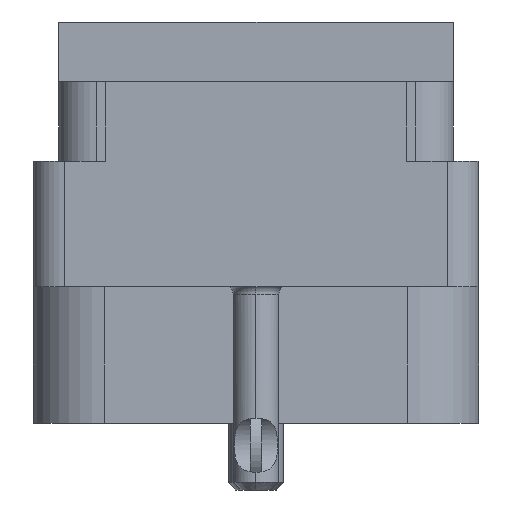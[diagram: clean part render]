
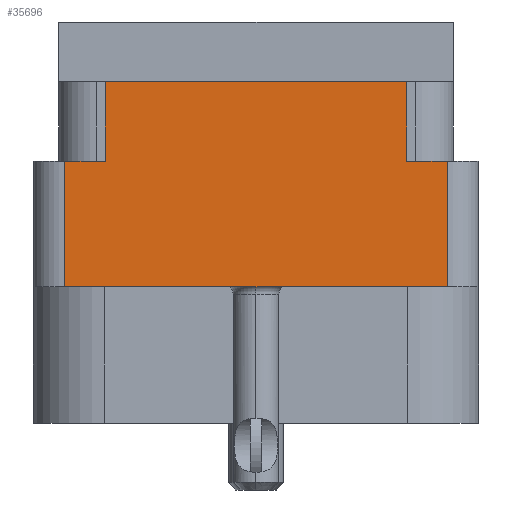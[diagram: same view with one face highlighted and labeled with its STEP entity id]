
A CAD part, left-side view. The second image highlights one B-rep face of the part: STEP entity #35696.
In plain terms, the highlighted planar face has unit normal (-1, 0, 0).
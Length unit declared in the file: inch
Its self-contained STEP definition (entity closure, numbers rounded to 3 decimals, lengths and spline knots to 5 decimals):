
#318 = DIRECTION ( 'NONE',  ( 0., -1., 0. ) ) ;
#1235 = PLANE ( 'NONE',  #37064 ) ;
#1629 = VERTEX_POINT ( 'NONE', #34674 ) ;
#1836 = DIRECTION ( 'NONE',  ( 0., 0., 1. ) ) ;
#2263 = DIRECTION ( 'NONE',  ( 0., -1., 0. ) ) ;
#3918 = ORIENTED_EDGE ( 'NONE', *, *, #47115, .F. ) ;
#5083 = CARTESIAN_POINT ( 'NONE',  ( -1.2955, 0.376, -0.274 ) ) ;
#5704 = CARTESIAN_POINT ( 'NONE',  ( -1.2955, -0.296, -0.274 ) ) ;
#7746 = LINE ( 'NONE', #5704, #24823 ) ;
#7964 = LINE ( 'NONE', #19664, #28378 ) ;
#8555 = CARTESIAN_POINT ( 'NONE',  ( -1.2955, 0., -0.274 ) ) ;
#11412 = CARTESIAN_POINT ( 'NONE',  ( -1.2955, -0.376, -0.274 ) ) ;
#11689 = ORIENTED_EDGE ( 'NONE', *, *, #15598, .T. ) ;
#11895 = VERTEX_POINT ( 'NONE', #47267 ) ;
#12795 = VECTOR ( 'NONE', #50683, 39.37008 ) ;
#13521 = DIRECTION ( 'NONE',  ( 0., 0., 1. ) ) ;
#14564 = ORIENTED_EDGE ( 'NONE', *, *, #44492, .F. ) ;
#14705 = VERTEX_POINT ( 'NONE', #22214 ) ;
#15155 = VERTEX_POINT ( 'NONE', #5083 ) ;
#15598 = EDGE_CURVE ( 'NONE', #14705, #17348, #41476, .T. ) ;
#16089 = ORIENTED_EDGE ( 'NONE', *, *, #51833, .T. ) ;
#17348 = VERTEX_POINT ( 'NONE', #11412 ) ;
#18699 = CARTESIAN_POINT ( 'NONE',  ( -1.2955, 0.296, -0.274 ) ) ;
#19311 = EDGE_CURVE ( 'NONE', #35578, #11895, #7746, .T. ) ;
#19664 = CARTESIAN_POINT ( 'NONE',  ( -1.2955, 0., -0.52 ) ) ;
#20456 = EDGE_CURVE ( 'NONE', #15155, #1629, #37213, .T. ) ;
#21814 = CARTESIAN_POINT ( 'NONE',  ( -1.2955, -0.438, -0.789 ) ) ;
#22182 = CARTESIAN_POINT ( 'NONE',  ( -1.2955, 0.376, -0.52 ) ) ;
#22214 = CARTESIAN_POINT ( 'NONE',  ( -1.2955, -0.376, -0.52 ) ) ;
#24001 = LINE ( 'NONE', #42652, #12795 ) ;
#24146 = EDGE_CURVE ( 'NONE', #1629, #36001, #32335, .T. ) ;
#24823 = VECTOR ( 'NONE', #1836, 39.37008 ) ;
#26041 = DIRECTION ( 'NONE',  ( -1., 0., 0. ) ) ;
#28032 = CARTESIAN_POINT ( 'NONE',  ( -1.2955, 0.296, -0.117 ) ) ;
#28337 = CARTESIAN_POINT ( 'NONE',  ( -1.2955, -0.376, -0.789 ) ) ;
#28378 = VECTOR ( 'NONE', #32529, 39.37008 ) ;
#28864 = ORIENTED_EDGE ( 'NONE', *, *, #19311, .T. ) ;
#29723 = VECTOR ( 'NONE', #48146, 39.37008 ) ;
#31559 = VERTEX_POINT ( 'NONE', #22182 ) ;
#32335 = LINE ( 'NONE', #18699, #29723 ) ;
#32529 = DIRECTION ( 'NONE',  ( 0., 1., 0. ) ) ;
#33266 = LINE ( 'NONE', #41477, #53432 ) ;
#34674 = CARTESIAN_POINT ( 'NONE',  ( -1.2955, 0.296, -0.274 ) ) ;
#34977 = LINE ( 'NONE', #8555, #39547 ) ;
#35578 = VERTEX_POINT ( 'NONE', #45560 ) ;
#35662 = FACE_OUTER_BOUND ( 'NONE', #41168, .T. ) ;
#35696 = ADVANCED_FACE ( 'NONE', ( #35662 ), #1235, .T. ) ;
#35866 = CARTESIAN_POINT ( 'NONE',  ( -1.2955, 0., -0.274 ) ) ;
#36001 = VERTEX_POINT ( 'NONE', #28032 ) ;
#36189 = ORIENTED_EDGE ( 'NONE', *, *, #20456, .F. ) ;
#36593 = DIRECTION ( 'NONE',  ( 0., 0., 1. ) ) ;
#36616 = EDGE_CURVE ( 'NONE', #14705, #31559, #7964, .T. ) ;
#37064 = AXIS2_PLACEMENT_3D ( 'NONE', #21814, #26041, #13521 ) ;
#37213 = LINE ( 'NONE', #35866, #46947 ) ;
#39547 = VECTOR ( 'NONE', #318, 39.37008 ) ;
#40842 = VECTOR ( 'NONE', #36593, 39.37008 ) ;
#41168 = EDGE_LOOP ( 'NONE', ( #36189, #16089, #49606, #11689, #3918, #28864, #14564, #53272 ) ) ;
#41284 = DIRECTION ( 'NONE',  ( 0., 0., -1. ) ) ;
#41476 = LINE ( 'NONE', #28337, #40842 ) ;
#41477 = CARTESIAN_POINT ( 'NONE',  ( -1.2955, 0.376, -0.789 ) ) ;
#42652 = CARTESIAN_POINT ( 'NONE',  ( -1.2955, 0.438, -0.117 ) ) ;
#44492 = EDGE_CURVE ( 'NONE', #36001, #11895, #24001, .T. ) ;
#45560 = CARTESIAN_POINT ( 'NONE',  ( -1.2955, -0.296, -0.274 ) ) ;
#46947 = VECTOR ( 'NONE', #2263, 39.37008 ) ;
#47115 = EDGE_CURVE ( 'NONE', #35578, #17348, #34977, .T. ) ;
#47267 = CARTESIAN_POINT ( 'NONE',  ( -1.2955, -0.296, -0.117 ) ) ;
#48146 = DIRECTION ( 'NONE',  ( 0., 0., 1. ) ) ;
#49606 = ORIENTED_EDGE ( 'NONE', *, *, #36616, .F. ) ;
#50683 = DIRECTION ( 'NONE',  ( 0., -1., 0. ) ) ;
#51833 = EDGE_CURVE ( 'NONE', #15155, #31559, #33266, .T. ) ;
#53272 = ORIENTED_EDGE ( 'NONE', *, *, #24146, .F. ) ;
#53432 = VECTOR ( 'NONE', #41284, 39.37008 ) ;
